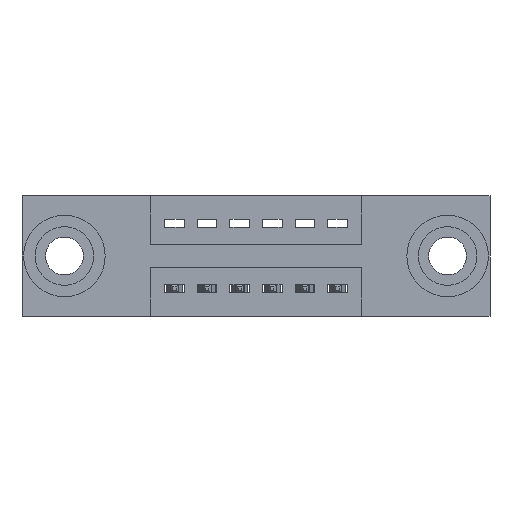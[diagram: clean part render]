
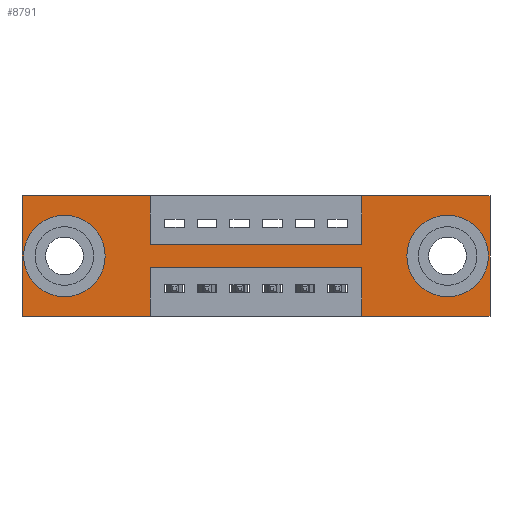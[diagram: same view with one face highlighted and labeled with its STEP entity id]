
A CAD part, front view. The second image highlights one B-rep face of the part: STEP entity #8791.
In plain terms, the highlighted planar face has unit normal (0, -1, 0).
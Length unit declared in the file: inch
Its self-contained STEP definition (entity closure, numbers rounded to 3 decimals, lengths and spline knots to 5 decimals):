
#72 = LINE ( 'NONE', #9753, #8225 ) ;
#250 = VERTEX_POINT ( 'NONE', #435 ) ;
#322 = CARTESIAN_POINT ( 'NONE',  ( 0.3925, 0., -0.15 ) ) ;
#435 = CARTESIAN_POINT ( 'NONE',  ( 0., 0., 0. ) ) ;
#468 = DIRECTION ( 'NONE',  ( 1., 0., 0. ) ) ;
#655 = EDGE_CURVE ( 'NONE', #8559, #9873, #1194, .T. ) ;
#677 = LINE ( 'NONE', #2872, #4580 ) ;
#710 = CARTESIAN_POINT ( 'NONE',  ( 1.305, 0., -0.263 ) ) ;
#819 = LINE ( 'NONE', #7440, #4359 ) ;
#860 = EDGE_CURVE ( 'NONE', #6592, #2805, #72, .T. ) ;
#901 = CARTESIAN_POINT ( 'NONE',  ( 1.0425, 0., -0.22 ) ) ;
#1172 = EDGE_CURVE ( 'NONE', #4526, #8962, #8573, .T. ) ;
#1194 = LINE ( 'NONE', #4231, #6904 ) ;
#1284 = CARTESIAN_POINT ( 'NONE',  ( 0., 0., 0. ) ) ;
#1451 = DIRECTION ( 'NONE',  ( 0., 0., -1. ) ) ;
#1529 = DIRECTION ( 'NONE',  ( 0., 0., 1. ) ) ;
#1574 = VECTOR ( 'NONE', #5700, 39.37008 ) ;
#1575 = AXIS2_PLACEMENT_3D ( 'NONE', #7840, #3167, #1529 ) ;
#1577 = CIRCLE ( 'NONE', #2464, 0.078 ) ;
#1604 = ORIENTED_EDGE ( 'NONE', *, *, #5736, .F. ) ;
#1662 = CARTESIAN_POINT ( 'NONE',  ( 1.305, 0., -0.185 ) ) ;
#1799 = VECTOR ( 'NONE', #468, 39.37008 ) ;
#1822 = CARTESIAN_POINT ( 'NONE',  ( 1.435, 0., -0.37 ) ) ;
#1899 = CARTESIAN_POINT ( 'NONE',  ( 0., 0., 0. ) ) ;
#1932 = DIRECTION ( 'NONE',  ( 0., 0., 1. ) ) ;
#2105 = DIRECTION ( 'NONE',  ( -1., 0., 0. ) ) ;
#2197 = LINE ( 'NONE', #9857, #9985 ) ;
#2211 = ORIENTED_EDGE ( 'NONE', *, *, #7885, .F. ) ;
#2231 = VERTEX_POINT ( 'NONE', #710 ) ;
#2247 = CARTESIAN_POINT ( 'NONE',  ( 1.305, 0., -0.107 ) ) ;
#2271 = EDGE_CURVE ( 'NONE', #2231, #6297, #5831, .T. ) ;
#2315 = CIRCLE ( 'NONE', #9758, 0.078 ) ;
#2416 = FACE_BOUND ( 'NONE', #5270, .T. ) ;
#2424 = VECTOR ( 'NONE', #9863, 39.37008 ) ;
#2464 = AXIS2_PLACEMENT_3D ( 'NONE', #7296, #3489, #9689 ) ;
#2623 = ORIENTED_EDGE ( 'NONE', *, *, #1172, .F. ) ;
#2624 = VERTEX_POINT ( 'NONE', #6578 ) ;
#2654 = DIRECTION ( 'NONE',  ( 0., 0., -1. ) ) ;
#2805 = VERTEX_POINT ( 'NONE', #5299 ) ;
#2872 = CARTESIAN_POINT ( 'NONE',  ( 1.0425, 0., -0.37 ) ) ;
#2891 = CARTESIAN_POINT ( 'NONE',  ( 0., 0., -0.37 ) ) ;
#3167 = DIRECTION ( 'NONE',  ( 0., 1., 0. ) ) ;
#3268 = VERTEX_POINT ( 'NONE', #1822 ) ;
#3320 = EDGE_CURVE ( 'NONE', #9873, #6592, #6962, .T. ) ;
#3451 = VERTEX_POINT ( 'NONE', #6793 ) ;
#3489 = DIRECTION ( 'NONE',  ( 0., 1., 0. ) ) ;
#3650 = PLANE ( 'NONE',  #6735 ) ;
#3656 = EDGE_CURVE ( 'NONE', #250, #8559, #5491, .T. ) ;
#3667 = EDGE_CURVE ( 'NONE', #2805, #6155, #5721, .T. ) ;
#3909 = CARTESIAN_POINT ( 'NONE',  ( 1.305, 0., -0.185 ) ) ;
#4078 = CARTESIAN_POINT ( 'NONE',  ( 0.3925, 0., 0. ) ) ;
#4089 = CARTESIAN_POINT ( 'NONE',  ( 0.3925, 0., -0.22 ) ) ;
#4099 = CARTESIAN_POINT ( 'NONE',  ( 0.13, 0., -0.107 ) ) ;
#4137 = LINE ( 'NONE', #1899, #1574 ) ;
#4231 = CARTESIAN_POINT ( 'NONE',  ( 0.3925, 0., 0. ) ) ;
#4359 = VECTOR ( 'NONE', #2654, 39.37008 ) ;
#4422 = DIRECTION ( 'NONE',  ( 0., 0., 1. ) ) ;
#4526 = VERTEX_POINT ( 'NONE', #4719 ) ;
#4561 = EDGE_CURVE ( 'NONE', #6297, #2231, #2315, .T. ) ;
#4565 = DIRECTION ( 'NONE',  ( 0., 0., -1. ) ) ;
#4580 = VECTOR ( 'NONE', #4422, 39.37008 ) ;
#4719 = CARTESIAN_POINT ( 'NONE',  ( 0.3925, 0., -0.37 ) ) ;
#4790 = VECTOR ( 'NONE', #7417, 39.37008 ) ;
#4847 = DIRECTION ( 'NONE',  ( 0., 0., -1. ) ) ;
#4986 = VECTOR ( 'NONE', #4565, 39.37008 ) ;
#5112 = LINE ( 'NONE', #10036, #4986 ) ;
#5253 = ORIENTED_EDGE ( 'NONE', *, *, #3656, .F. ) ;
#5270 = EDGE_LOOP ( 'NONE', ( #9537, #5302 ) ) ;
#5280 = DIRECTION ( 'NONE',  ( -1., 0., 0. ) ) ;
#5299 = CARTESIAN_POINT ( 'NONE',  ( 1.0425, 0., 0. ) ) ;
#5302 = ORIENTED_EDGE ( 'NONE', *, *, #2271, .T. ) ;
#5308 = CARTESIAN_POINT ( 'NONE',  ( 1.0425, 0., -0.15 ) ) ;
#5491 = LINE ( 'NONE', #9594, #2424 ) ;
#5619 = VERTEX_POINT ( 'NONE', #5952 ) ;
#5700 = DIRECTION ( 'NONE',  ( 0., 0., 1. ) ) ;
#5721 = LINE ( 'NONE', #1284, #1799 ) ;
#5736 = EDGE_CURVE ( 'NONE', #6155, #3268, #5112, .T. ) ;
#5828 = ORIENTED_EDGE ( 'NONE', *, *, #3667, .F. ) ;
#5831 = CIRCLE ( 'NONE', #7288, 0.078 ) ;
#5882 = EDGE_LOOP ( 'NONE', ( #9832, #9209 ) ) ;
#5889 = ORIENTED_EDGE ( 'NONE', *, *, #860, .F. ) ;
#5952 = CARTESIAN_POINT ( 'NONE',  ( 0.3925, 0., -0.22 ) ) ;
#6043 = CARTESIAN_POINT ( 'NONE',  ( 0.3925, 0., -0.15 ) ) ;
#6155 = VERTEX_POINT ( 'NONE', #9324 ) ;
#6297 = VERTEX_POINT ( 'NONE', #2247 ) ;
#6329 = DIRECTION ( 'NONE',  ( -1., 0., 0. ) ) ;
#6405 = EDGE_CURVE ( 'NONE', #9674, #3451, #1577, .T. ) ;
#6578 = CARTESIAN_POINT ( 'NONE',  ( 1.0425, 0., -0.37 ) ) ;
#6592 = VERTEX_POINT ( 'NONE', #5308 ) ;
#6647 = EDGE_CURVE ( 'NONE', #2624, #8189, #677, .T. ) ;
#6735 = AXIS2_PLACEMENT_3D ( 'NONE', #2891, #9072, #8974 ) ;
#6793 = CARTESIAN_POINT ( 'NONE',  ( 0.13, 0., -0.263 ) ) ;
#6904 = VECTOR ( 'NONE', #9582, 39.37008 ) ;
#6962 = LINE ( 'NONE', #322, #4790 ) ;
#7181 = EDGE_CURVE ( 'NONE', #3268, #2624, #2197, .T. ) ;
#7236 = VECTOR ( 'NONE', #6329, 39.37008 ) ;
#7280 = ORIENTED_EDGE ( 'NONE', *, *, #655, .F. ) ;
#7288 = AXIS2_PLACEMENT_3D ( 'NONE', #3909, #7792, #1451 ) ;
#7296 = CARTESIAN_POINT ( 'NONE',  ( 0.13, 0., -0.185 ) ) ;
#7358 = ORIENTED_EDGE ( 'NONE', *, *, #7507, .F. ) ;
#7417 = DIRECTION ( 'NONE',  ( 1., 0., 0. ) ) ;
#7440 = CARTESIAN_POINT ( 'NONE',  ( 0.3925, 0., -0.37 ) ) ;
#7507 = EDGE_CURVE ( 'NONE', #5619, #4526, #819, .T. ) ;
#7611 = EDGE_LOOP ( 'NONE', ( #7358, #7643, #9063, #8801, #1604, #5828, #5889, #9089, #7280, #5253, #2211, #2623 ) ) ;
#7643 = ORIENTED_EDGE ( 'NONE', *, *, #8611, .F. ) ;
#7768 = CARTESIAN_POINT ( 'NONE',  ( 0., 0., -0.37 ) ) ;
#7792 = DIRECTION ( 'NONE',  ( 0., 1., 0. ) ) ;
#7840 = CARTESIAN_POINT ( 'NONE',  ( 0.13, 0., -0.185 ) ) ;
#7885 = EDGE_CURVE ( 'NONE', #8962, #250, #4137, .T. ) ;
#7986 = EDGE_CURVE ( 'NONE', #3451, #9674, #8034, .T. ) ;
#8034 = CIRCLE ( 'NONE', #1575, 0.078 ) ;
#8164 = VECTOR ( 'NONE', #5280, 39.37008 ) ;
#8189 = VERTEX_POINT ( 'NONE', #901 ) ;
#8225 = VECTOR ( 'NONE', #1932, 39.37008 ) ;
#8559 = VERTEX_POINT ( 'NONE', #4078 ) ;
#8573 = LINE ( 'NONE', #9406, #7236 ) ;
#8611 = EDGE_CURVE ( 'NONE', #8189, #5619, #9974, .T. ) ;
#8791 = ADVANCED_FACE ( 'NONE', ( #2416, #9605, #9125 ), #3650, .T. ) ;
#8801 = ORIENTED_EDGE ( 'NONE', *, *, #7181, .F. ) ;
#8962 = VERTEX_POINT ( 'NONE', #7768 ) ;
#8974 = DIRECTION ( 'NONE',  ( 0., 0., -1. ) ) ;
#9063 = ORIENTED_EDGE ( 'NONE', *, *, #6647, .F. ) ;
#9072 = DIRECTION ( 'NONE',  ( 0., -1., 0. ) ) ;
#9089 = ORIENTED_EDGE ( 'NONE', *, *, #3320, .F. ) ;
#9125 = FACE_OUTER_BOUND ( 'NONE', #7611, .T. ) ;
#9209 = ORIENTED_EDGE ( 'NONE', *, *, #7986, .T. ) ;
#9324 = CARTESIAN_POINT ( 'NONE',  ( 1.435, 0., 0. ) ) ;
#9406 = CARTESIAN_POINT ( 'NONE',  ( 0., 0., -0.37 ) ) ;
#9442 = DIRECTION ( 'NONE',  ( 0., 1., 0. ) ) ;
#9537 = ORIENTED_EDGE ( 'NONE', *, *, #4561, .T. ) ;
#9582 = DIRECTION ( 'NONE',  ( 0., 0., -1. ) ) ;
#9594 = CARTESIAN_POINT ( 'NONE',  ( 0., 0., 0. ) ) ;
#9605 = FACE_BOUND ( 'NONE', #5882, .T. ) ;
#9674 = VERTEX_POINT ( 'NONE', #4099 ) ;
#9689 = DIRECTION ( 'NONE',  ( 0., 0., 1. ) ) ;
#9753 = CARTESIAN_POINT ( 'NONE',  ( 1.0425, 0., 0. ) ) ;
#9758 = AXIS2_PLACEMENT_3D ( 'NONE', #1662, #9442, #4847 ) ;
#9832 = ORIENTED_EDGE ( 'NONE', *, *, #6405, .T. ) ;
#9857 = CARTESIAN_POINT ( 'NONE',  ( 0., 0., -0.37 ) ) ;
#9863 = DIRECTION ( 'NONE',  ( 1., 0., 0. ) ) ;
#9873 = VERTEX_POINT ( 'NONE', #6043 ) ;
#9974 = LINE ( 'NONE', #4089, #8164 ) ;
#9985 = VECTOR ( 'NONE', #2105, 39.37008 ) ;
#10036 = CARTESIAN_POINT ( 'NONE',  ( 1.435, 0., 0. ) ) ;
